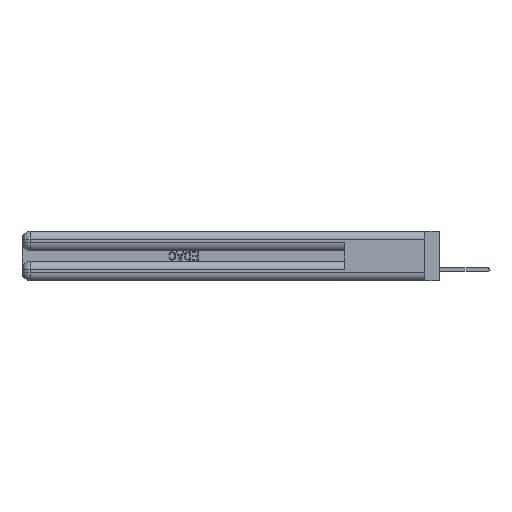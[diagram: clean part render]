
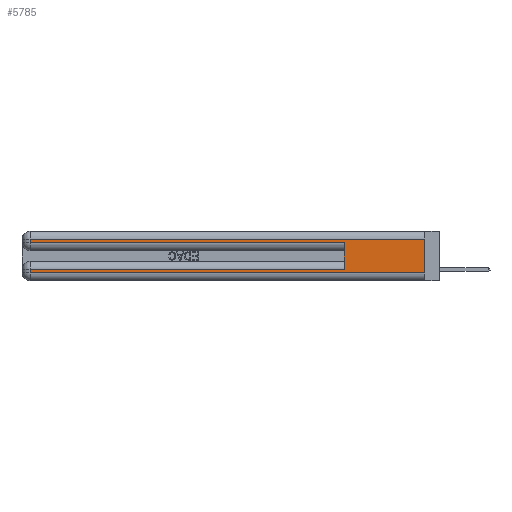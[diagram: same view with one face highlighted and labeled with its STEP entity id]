
A CAD part, left-side view. The second image highlights one B-rep face of the part: STEP entity #5785.
In plain terms, the highlighted planar face has unit normal (-1, 0, 0).
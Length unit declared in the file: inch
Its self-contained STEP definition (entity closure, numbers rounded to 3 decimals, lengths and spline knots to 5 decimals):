
#558 = VECTOR ( 'NONE', #33028, 39.37008 ) ;
#818 = EDGE_CURVE ( 'NONE', #48304, #10475, #24753, .T. ) ;
#2427 = CARTESIAN_POINT ( 'NONE',  ( 0., 0., 0.31 ) ) ;
#2662 = CARTESIAN_POINT ( 'NONE',  ( 0., 2.94, 0.285 ) ) ;
#4026 = CARTESIAN_POINT ( 'NONE',  ( 0., 0.6, 0.145 ) ) ;
#5785 = ADVANCED_FACE ( 'NONE', ( #48063 ), #46423, .F. ) ;
#6266 = ORIENTED_EDGE ( 'NONE', *, *, #7482, .T. ) ;
#7482 = EDGE_CURVE ( 'NONE', #36887, #18542, #35702, .T. ) ;
#7768 = DIRECTION ( 'NONE',  ( 0., 1., 0. ) ) ;
#9757 = VERTEX_POINT ( 'NONE', #35547 ) ;
#9912 = EDGE_CURVE ( 'NONE', #14045, #48404, #32857, .T. ) ;
#10475 = VERTEX_POINT ( 'NONE', #14531 ) ;
#10788 = ORIENTED_EDGE ( 'NONE', *, *, #9912, .T. ) ;
#11279 = CARTESIAN_POINT ( 'NONE',  ( 0., 0.6, 0.285 ) ) ;
#11540 = DIRECTION ( 'NONE',  ( 0., 0., -1. ) ) ;
#12691 = DIRECTION ( 'NONE',  ( 0., -1., 0. ) ) ;
#14045 = VERTEX_POINT ( 'NONE', #49795 ) ;
#14531 = CARTESIAN_POINT ( 'NONE',  ( 0., 0., 0.06 ) ) ;
#15009 = VECTOR ( 'NONE', #17012, 39.37008 ) ;
#15133 = VECTOR ( 'NONE', #34724, 39.37008 ) ;
#17012 = DIRECTION ( 'NONE',  ( 0., 0., 1. ) ) ;
#17588 = LINE ( 'NONE', #36605, #35142 ) ;
#17914 = ORIENTED_EDGE ( 'NONE', *, *, #30068, .T. ) ;
#18029 = EDGE_CURVE ( 'NONE', #9757, #14045, #17588, .T. ) ;
#18542 = VERTEX_POINT ( 'NONE', #2662 ) ;
#18544 = CARTESIAN_POINT ( 'NONE',  ( 0., 0., 0.37 ) ) ;
#18579 = VERTEX_POINT ( 'NONE', #11279 ) ;
#20033 = ORIENTED_EDGE ( 'NONE', *, *, #36856, .T. ) ;
#24023 = EDGE_LOOP ( 'NONE', ( #50271, #36904, #6266, #20033, #43980, #33863, #10788, #17914 ) ) ;
#24753 = LINE ( 'NONE', #18544, #45521 ) ;
#27174 = CARTESIAN_POINT ( 'NONE',  ( 0., 2.94, 0.37 ) ) ;
#29944 = LINE ( 'NONE', #44922, #49389 ) ;
#29949 = DIRECTION ( 'NONE',  ( 0., 0., -1. ) ) ;
#30068 = EDGE_CURVE ( 'NONE', #48404, #10475, #29944, .T. ) ;
#30366 = CARTESIAN_POINT ( 'NONE',  ( 0., 2.94, 0.37 ) ) ;
#32703 = CARTESIAN_POINT ( 'NONE',  ( 0., 0., 0.285 ) ) ;
#32857 = LINE ( 'NONE', #30366, #45043 ) ;
#33028 = DIRECTION ( 'NONE',  ( 0., -1., 0. ) ) ;
#33863 = ORIENTED_EDGE ( 'NONE', *, *, #18029, .T. ) ;
#34724 = DIRECTION ( 'NONE',  ( 0., 0., -1. ) ) ;
#34747 = LINE ( 'NONE', #34822, #37733 ) ;
#34766 = EDGE_CURVE ( 'NONE', #9757, #18579, #47242, .T. ) ;
#34822 = CARTESIAN_POINT ( 'NONE',  ( 0., 0., 0.31 ) ) ;
#34991 = CARTESIAN_POINT ( 'NONE',  ( 0., 2.94, 0.06 ) ) ;
#35142 = VECTOR ( 'NONE', #42335, 39.37008 ) ;
#35547 = CARTESIAN_POINT ( 'NONE',  ( 0., 0.6, 0.085 ) ) ;
#35702 = LINE ( 'NONE', #27174, #15133 ) ;
#36605 = CARTESIAN_POINT ( 'NONE',  ( 0., 0., 0.085 ) ) ;
#36856 = EDGE_CURVE ( 'NONE', #18542, #18579, #44613, .T. ) ;
#36887 = VERTEX_POINT ( 'NONE', #49043 ) ;
#36904 = ORIENTED_EDGE ( 'NONE', *, *, #37817, .T. ) ;
#37733 = VECTOR ( 'NONE', #7768, 39.37008 ) ;
#37817 = EDGE_CURVE ( 'NONE', #48304, #36887, #34747, .T. ) ;
#38381 = DIRECTION ( 'NONE',  ( 1., 0., 0. ) ) ;
#38726 = CARTESIAN_POINT ( 'NONE',  ( 0., 0., 0.37 ) ) ;
#42335 = DIRECTION ( 'NONE',  ( 0., 1., 0. ) ) ;
#42424 = DIRECTION ( 'NONE',  ( 0., 0., -1. ) ) ;
#43980 = ORIENTED_EDGE ( 'NONE', *, *, #34766, .F. ) ;
#44603 = AXIS2_PLACEMENT_3D ( 'NONE', #38726, #38381, #11540 ) ;
#44613 = LINE ( 'NONE', #32703, #558 ) ;
#44922 = CARTESIAN_POINT ( 'NONE',  ( 0., 0., 0.06 ) ) ;
#45043 = VECTOR ( 'NONE', #42424, 39.37008 ) ;
#45521 = VECTOR ( 'NONE', #29949, 39.37008 ) ;
#46423 = PLANE ( 'NONE',  #44603 ) ;
#47242 = LINE ( 'NONE', #4026, #15009 ) ;
#48063 = FACE_OUTER_BOUND ( 'NONE', #24023, .T. ) ;
#48304 = VERTEX_POINT ( 'NONE', #2427 ) ;
#48404 = VERTEX_POINT ( 'NONE', #34991 ) ;
#49043 = CARTESIAN_POINT ( 'NONE',  ( 0., 2.94, 0.31 ) ) ;
#49389 = VECTOR ( 'NONE', #12691, 39.37008 ) ;
#49795 = CARTESIAN_POINT ( 'NONE',  ( 0., 2.94, 0.085 ) ) ;
#50271 = ORIENTED_EDGE ( 'NONE', *, *, #818, .F. ) ;
